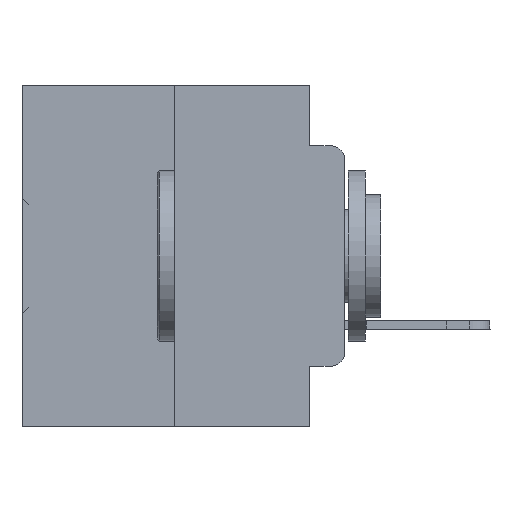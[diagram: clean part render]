
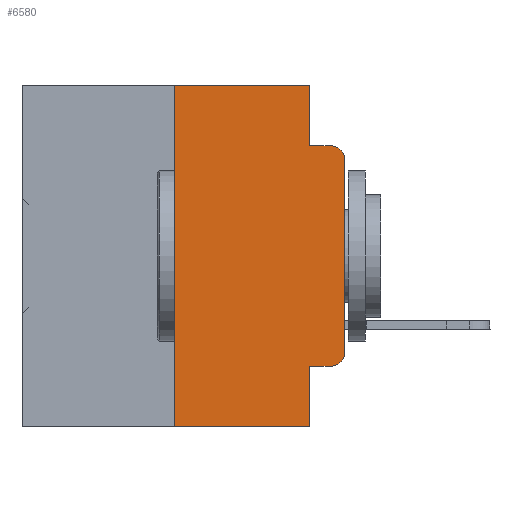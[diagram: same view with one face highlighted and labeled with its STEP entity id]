
A CAD part, left-side view. The second image highlights one B-rep face of the part: STEP entity #6580.
In plain terms, the highlighted planar face has unit normal (-1, 0, 0).
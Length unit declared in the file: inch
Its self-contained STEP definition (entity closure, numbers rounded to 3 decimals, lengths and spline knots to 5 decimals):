
#219 = CARTESIAN_POINT ( 'NONE',  ( 0., 0.051, -0.4115 ) ) ;
#342 = LINE ( 'NONE', #19918, #35140 ) ;
#2564 = LINE ( 'NONE', #14069, #27396 ) ;
#2947 = CARTESIAN_POINT ( 'NONE',  ( 0., 0.25, 0. ) ) ;
#2959 = ORIENTED_EDGE ( 'NONE', *, *, #12380, .F. ) ;
#3257 = CARTESIAN_POINT ( 'NONE',  ( 0., 0.25, -0.5 ) ) ;
#4562 = DIRECTION ( 'NONE',  ( 0., 0., -1. ) ) ;
#4701 = EDGE_CURVE ( 'NONE', #33760, #35126, #24105, .T. ) ;
#5054 = ORIENTED_EDGE ( 'NONE', *, *, #29640, .T. ) ;
#5090 = VECTOR ( 'NONE', #6035, 39.37008 ) ;
#5862 = VERTEX_POINT ( 'NONE', #27951 ) ;
#6035 = DIRECTION ( 'NONE',  ( 0., 0., -1. ) ) ;
#6422 = CARTESIAN_POINT ( 'NONE',  ( 0., 0.051, 0. ) ) ;
#6580 = ADVANCED_FACE ( 'NONE', ( #7028 ), #12297, .F. ) ;
#6800 = ORIENTED_EDGE ( 'NONE', *, *, #18675, .F. ) ;
#7028 = FACE_OUTER_BOUND ( 'NONE', #8993, .T. ) ;
#7449 = CARTESIAN_POINT ( 'NONE',  ( 0., 0.473, 0. ) ) ;
#7643 = VECTOR ( 'NONE', #12460, 39.37008 ) ;
#7822 = ORIENTED_EDGE ( 'NONE', *, *, #12734, .T. ) ;
#8113 = DIRECTION ( 'NONE',  ( 0., 0., 1. ) ) ;
#8577 = VECTOR ( 'NONE', #34960, 39.37008 ) ;
#8676 = LINE ( 'NONE', #28786, #5090 ) ;
#8885 = CARTESIAN_POINT ( 'NONE',  ( 0., 0.051, 0. ) ) ;
#8993 = EDGE_LOOP ( 'NONE', ( #15604, #5054, #2959, #19862, #32502, #6800, #24438, #12008, #18948, #7822 ) ) ;
#9305 = VERTEX_POINT ( 'NONE', #36565 ) ;
#9353 = VECTOR ( 'NONE', #8113, 39.37008 ) ;
#9542 = VERTEX_POINT ( 'NONE', #20404 ) ;
#9742 = AXIS2_PLACEMENT_3D ( 'NONE', #16236, #21307, #4562 ) ;
#12008 = ORIENTED_EDGE ( 'NONE', *, *, #19682, .F. ) ;
#12297 = PLANE ( 'NONE',  #16948 ) ;
#12380 = EDGE_CURVE ( 'NONE', #35126, #16261, #342, .T. ) ;
#12460 = DIRECTION ( 'NONE',  ( 0., 0., -1. ) ) ;
#12519 = VERTEX_POINT ( 'NONE', #20650 ) ;
#12734 = EDGE_CURVE ( 'NONE', #9305, #5862, #35801, .T. ) ;
#12903 = EDGE_CURVE ( 'NONE', #19222, #12519, #2564, .T. ) ;
#13901 = DIRECTION ( 'NONE',  ( 0., 0., 1. ) ) ;
#14069 = CARTESIAN_POINT ( 'NONE',  ( 0., 0.473, -0.5 ) ) ;
#14256 = LINE ( 'NONE', #2947, #32442 ) ;
#15274 = LINE ( 'NONE', #219, #8577 ) ;
#15461 = CARTESIAN_POINT ( 'NONE',  ( 0., 0.02, -0.0885 ) ) ;
#15604 = ORIENTED_EDGE ( 'NONE', *, *, #36850, .T. ) ;
#16236 = CARTESIAN_POINT ( 'NONE',  ( 0., 0.02, -0.1085 ) ) ;
#16261 = VERTEX_POINT ( 'NONE', #15461 ) ;
#16948 = AXIS2_PLACEMENT_3D ( 'NONE', #27128, #18126, #35185 ) ;
#17376 = VERTEX_POINT ( 'NONE', #31826 ) ;
#18126 = DIRECTION ( 'NONE',  ( 1., 0., 0. ) ) ;
#18675 = EDGE_CURVE ( 'NONE', #19222, #37076, #14256, .T. ) ;
#18929 = DIRECTION ( 'NONE',  ( 0., -1., 0. ) ) ;
#18948 = ORIENTED_EDGE ( 'NONE', *, *, #32601, .T. ) ;
#19156 = DIRECTION ( 'NONE',  ( -1., 0., 0. ) ) ;
#19222 = VERTEX_POINT ( 'NONE', #3257 ) ;
#19682 = EDGE_CURVE ( 'NONE', #9542, #12519, #8676, .T. ) ;
#19862 = ORIENTED_EDGE ( 'NONE', *, *, #4701, .F. ) ;
#19918 = CARTESIAN_POINT ( 'NONE',  ( 0., 0.051, -0.0885 ) ) ;
#20404 = CARTESIAN_POINT ( 'NONE',  ( 0., 0.051, -0.4115 ) ) ;
#20650 = CARTESIAN_POINT ( 'NONE',  ( 0., 0.051, -0.5 ) ) ;
#21307 = DIRECTION ( 'NONE',  ( -1., 0., 0. ) ) ;
#22152 = DIRECTION ( 'NONE',  ( 0., 0., -1. ) ) ;
#22412 = CARTESIAN_POINT ( 'NONE',  ( 0., 0., 0. ) ) ;
#23805 = AXIS2_PLACEMENT_3D ( 'NONE', #36214, #19156, #22152 ) ;
#24105 = LINE ( 'NONE', #6422, #7643 ) ;
#24438 = ORIENTED_EDGE ( 'NONE', *, *, #12903, .T. ) ;
#25491 = DIRECTION ( 'NONE',  ( 0., -1., 0. ) ) ;
#25909 = DIRECTION ( 'NONE',  ( 0., -1., 0. ) ) ;
#26134 = LINE ( 'NONE', #22412, #9353 ) ;
#27128 = CARTESIAN_POINT ( 'NONE',  ( 0., 0.473, 0. ) ) ;
#27396 = VECTOR ( 'NONE', #25491, 39.37008 ) ;
#27951 = CARTESIAN_POINT ( 'NONE',  ( 0., 0., -0.3915 ) ) ;
#28260 = CARTESIAN_POINT ( 'NONE',  ( 0., 0.051, -0.0885 ) ) ;
#28786 = CARTESIAN_POINT ( 'NONE',  ( 0., 0.051, 0. ) ) ;
#29552 = VECTOR ( 'NONE', #18929, 39.37008 ) ;
#29640 = EDGE_CURVE ( 'NONE', #17376, #16261, #34327, .T. ) ;
#30696 = EDGE_CURVE ( 'NONE', #37076, #33760, #33186, .T. ) ;
#31826 = CARTESIAN_POINT ( 'NONE',  ( 0., 0., -0.1085 ) ) ;
#32442 = VECTOR ( 'NONE', #13901, 39.37008 ) ;
#32502 = ORIENTED_EDGE ( 'NONE', *, *, #30696, .F. ) ;
#32601 = EDGE_CURVE ( 'NONE', #9542, #9305, #15274, .T. ) ;
#33186 = LINE ( 'NONE', #7449, #29552 ) ;
#33636 = CARTESIAN_POINT ( 'NONE',  ( 0., 0.25, 0. ) ) ;
#33760 = VERTEX_POINT ( 'NONE', #8885 ) ;
#34327 = CIRCLE ( 'NONE', #9742, 0.02 ) ;
#34960 = DIRECTION ( 'NONE',  ( 0., -1., 0. ) ) ;
#35126 = VERTEX_POINT ( 'NONE', #28260 ) ;
#35140 = VECTOR ( 'NONE', #25909, 39.37008 ) ;
#35185 = DIRECTION ( 'NONE',  ( 0., 0., -1. ) ) ;
#35801 = CIRCLE ( 'NONE', #23805, 0.02 ) ;
#36214 = CARTESIAN_POINT ( 'NONE',  ( 0., 0.02, -0.3915 ) ) ;
#36565 = CARTESIAN_POINT ( 'NONE',  ( 0., 0.02, -0.4115 ) ) ;
#36850 = EDGE_CURVE ( 'NONE', #5862, #17376, #26134, .T. ) ;
#37076 = VERTEX_POINT ( 'NONE', #33636 ) ;
